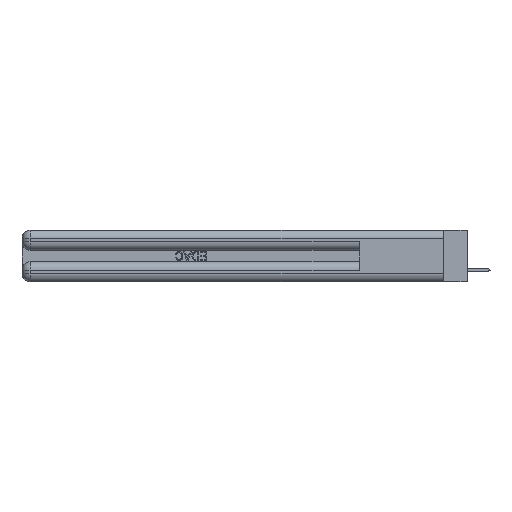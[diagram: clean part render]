
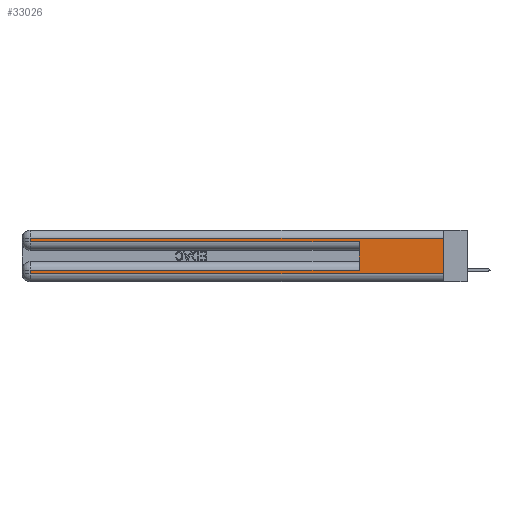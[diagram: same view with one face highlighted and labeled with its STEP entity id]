
A CAD part, left-side view. The second image highlights one B-rep face of the part: STEP entity #33026.
In plain terms, the highlighted planar face has unit normal (-1, 0, 0).
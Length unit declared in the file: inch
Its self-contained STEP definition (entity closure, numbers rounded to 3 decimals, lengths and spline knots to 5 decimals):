
#1491 = LINE ( 'NONE', #26850, #6640 ) ;
#1759 = VECTOR ( 'NONE', #35572, 39.37008 ) ;
#1948 = PLANE ( 'NONE',  #38433 ) ;
#2519 = CARTESIAN_POINT ( 'NONE',  ( 0., 0., 0.085 ) ) ;
#2810 = LINE ( 'NONE', #25639, #27108 ) ;
#3562 = LINE ( 'NONE', #5697, #33134 ) ;
#4114 = DIRECTION ( 'NONE',  ( 0., 0., 1. ) ) ;
#5601 = EDGE_CURVE ( 'NONE', #31272, #25331, #7984, .T. ) ;
#5628 = EDGE_CURVE ( 'NONE', #37248, #38043, #2810, .T. ) ;
#5697 = CARTESIAN_POINT ( 'NONE',  ( 0., 0., 0.06 ) ) ;
#6051 = VERTEX_POINT ( 'NONE', #39051 ) ;
#6640 = VECTOR ( 'NONE', #4114, 39.37008 ) ;
#6730 = EDGE_CURVE ( 'NONE', #6051, #37248, #33659, .T. ) ;
#6940 = DIRECTION ( 'NONE',  ( 0., 1., 0. ) ) ;
#7886 = ORIENTED_EDGE ( 'NONE', *, *, #6730, .T. ) ;
#7984 = LINE ( 'NONE', #9448, #8955 ) ;
#8273 = VECTOR ( 'NONE', #6940, 39.37008 ) ;
#8595 = LINE ( 'NONE', #11062, #35379 ) ;
#8677 = DIRECTION ( 'NONE',  ( 0., -1., 0. ) ) ;
#8955 = VECTOR ( 'NONE', #33991, 39.37008 ) ;
#9122 = LINE ( 'NONE', #35905, #18657 ) ;
#9229 = LINE ( 'NONE', #31064, #8273 ) ;
#9448 = CARTESIAN_POINT ( 'NONE',  ( 0., 0., 0.37 ) ) ;
#9706 = CARTESIAN_POINT ( 'NONE',  ( 0., 2.94, 0.085 ) ) ;
#11062 = CARTESIAN_POINT ( 'NONE',  ( 0., 2.94, 0.37 ) ) ;
#11258 = EDGE_CURVE ( 'NONE', #6051, #33572, #1491, .T. ) ;
#11816 = DIRECTION ( 'NONE',  ( 0., -1., 0. ) ) ;
#13174 = EDGE_LOOP ( 'NONE', ( #20908, #32085, #33110, #25482, #14315, #7886, #21360, #37921 ) ) ;
#14153 = DIRECTION ( 'NONE',  ( 0., 0., -1. ) ) ;
#14292 = DIRECTION ( 'NONE',  ( 0., 0., -1. ) ) ;
#14315 = ORIENTED_EDGE ( 'NONE', *, *, #11258, .F. ) ;
#14562 = DIRECTION ( 'NONE',  ( 1., 0., 0. ) ) ;
#16711 = EDGE_CURVE ( 'NONE', #31272, #19961, #9229, .T. ) ;
#17459 = CARTESIAN_POINT ( 'NONE',  ( 0., 0., 0.37 ) ) ;
#18657 = VECTOR ( 'NONE', #8677, 39.37008 ) ;
#18689 = CARTESIAN_POINT ( 'NONE',  ( 0., 2.94, 0.31 ) ) ;
#19829 = CARTESIAN_POINT ( 'NONE',  ( 0., 0.6, 0.285 ) ) ;
#19961 = VERTEX_POINT ( 'NONE', #18689 ) ;
#20908 = ORIENTED_EDGE ( 'NONE', *, *, #5601, .F. ) ;
#21360 = ORIENTED_EDGE ( 'NONE', *, *, #5628, .T. ) ;
#21852 = VERTEX_POINT ( 'NONE', #36206 ) ;
#25331 = VERTEX_POINT ( 'NONE', #32718 ) ;
#25414 = CARTESIAN_POINT ( 'NONE',  ( 0., 0., 0.31 ) ) ;
#25482 = ORIENTED_EDGE ( 'NONE', *, *, #35180, .T. ) ;
#25639 = CARTESIAN_POINT ( 'NONE',  ( 0., 2.94, 0.37 ) ) ;
#26850 = CARTESIAN_POINT ( 'NONE',  ( 0., 0.6, 0.145 ) ) ;
#27108 = VECTOR ( 'NONE', #28867, 39.37008 ) ;
#28274 = FACE_OUTER_BOUND ( 'NONE', #13174, .T. ) ;
#28867 = DIRECTION ( 'NONE',  ( 0., 0., -1. ) ) ;
#31064 = CARTESIAN_POINT ( 'NONE',  ( 0., 0., 0.31 ) ) ;
#31272 = VERTEX_POINT ( 'NONE', #25414 ) ;
#32085 = ORIENTED_EDGE ( 'NONE', *, *, #16711, .T. ) ;
#32718 = CARTESIAN_POINT ( 'NONE',  ( 0., 0., 0.06 ) ) ;
#33026 = ADVANCED_FACE ( 'NONE', ( #28274 ), #1948, .F. ) ;
#33110 = ORIENTED_EDGE ( 'NONE', *, *, #35721, .T. ) ;
#33134 = VECTOR ( 'NONE', #11816, 39.37008 ) ;
#33572 = VERTEX_POINT ( 'NONE', #19829 ) ;
#33659 = LINE ( 'NONE', #2519, #1759 ) ;
#33991 = DIRECTION ( 'NONE',  ( 0., 0., -1. ) ) ;
#34590 = CARTESIAN_POINT ( 'NONE',  ( 0., 2.94, 0.06 ) ) ;
#35180 = EDGE_CURVE ( 'NONE', #21852, #33572, #9122, .T. ) ;
#35379 = VECTOR ( 'NONE', #14153, 39.37008 ) ;
#35572 = DIRECTION ( 'NONE',  ( 0., 1., 0. ) ) ;
#35721 = EDGE_CURVE ( 'NONE', #19961, #21852, #8595, .T. ) ;
#35905 = CARTESIAN_POINT ( 'NONE',  ( 0., 0., 0.285 ) ) ;
#36206 = CARTESIAN_POINT ( 'NONE',  ( 0., 2.94, 0.285 ) ) ;
#37248 = VERTEX_POINT ( 'NONE', #9706 ) ;
#37921 = ORIENTED_EDGE ( 'NONE', *, *, #39102, .T. ) ;
#38043 = VERTEX_POINT ( 'NONE', #34590 ) ;
#38433 = AXIS2_PLACEMENT_3D ( 'NONE', #17459, #14562, #14292 ) ;
#39051 = CARTESIAN_POINT ( 'NONE',  ( 0., 0.6, 0.085 ) ) ;
#39102 = EDGE_CURVE ( 'NONE', #38043, #25331, #3562, .T. ) ;
